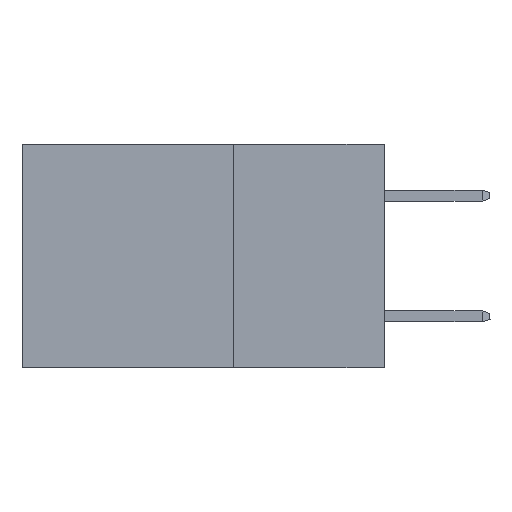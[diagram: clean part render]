
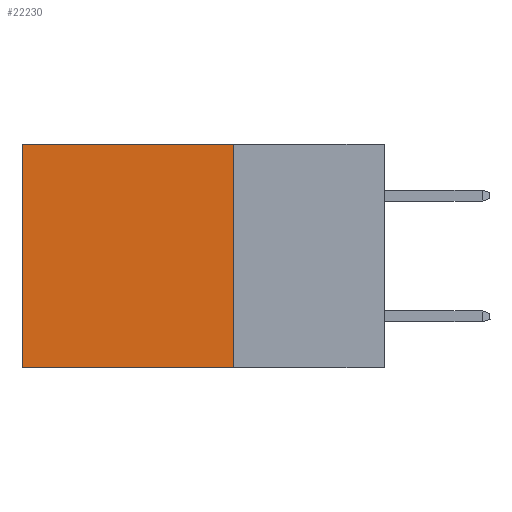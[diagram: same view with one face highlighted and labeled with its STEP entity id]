
A CAD part, left-side view. The second image highlights one B-rep face of the part: STEP entity #22230.
In plain terms, the highlighted planar face has unit normal (-1, 0, 0).
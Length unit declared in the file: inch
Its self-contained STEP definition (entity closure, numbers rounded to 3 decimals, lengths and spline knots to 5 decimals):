
#324 = CARTESIAN_POINT ( 'NONE',  ( 0.2615, 0.6, -0.37 ) ) ;
#365 = EDGE_LOOP ( 'NONE', ( #869, #15367, #24436, #25030 ) ) ;
#869 = ORIENTED_EDGE ( 'NONE', *, *, #14930, .T. ) ;
#1319 = CARTESIAN_POINT ( 'NONE',  ( 0.2615, 0.25, 0. ) ) ;
#2279 = LINE ( 'NONE', #3598, #12925 ) ;
#3598 = CARTESIAN_POINT ( 'NONE',  ( 0.2615, 0.25, -0.37 ) ) ;
#3680 = CARTESIAN_POINT ( 'NONE',  ( 0.2615, 0.25, 0. ) ) ;
#3895 = EDGE_CURVE ( 'NONE', #20038, #16957, #24164, .T. ) ;
#4118 = DIRECTION ( 'NONE',  ( 0., 0., -1. ) ) ;
#4498 = VECTOR ( 'NONE', #7657, 39.37008 ) ;
#4913 = CARTESIAN_POINT ( 'NONE',  ( 0.2615, 0.25, -0.37 ) ) ;
#5964 = VECTOR ( 'NONE', #4118, 39.37008 ) ;
#7657 = DIRECTION ( 'NONE',  ( 0., 1., 0. ) ) ;
#10347 = EDGE_CURVE ( 'NONE', #20038, #16766, #26864, .T. ) ;
#10681 = CARTESIAN_POINT ( 'NONE',  ( 0.2615, 0.25, -0.37 ) ) ;
#11601 = LINE ( 'NONE', #21002, #5964 ) ;
#12494 = DIRECTION ( 'NONE',  ( 0., 0., -1. ) ) ;
#12925 = VECTOR ( 'NONE', #22610, 39.37008 ) ;
#13458 = DIRECTION ( 'NONE',  ( 0., 0., -1. ) ) ;
#14129 = EDGE_CURVE ( 'NONE', #16957, #21756, #2279, .T. ) ;
#14930 = EDGE_CURVE ( 'NONE', #16766, #21756, #11601, .T. ) ;
#15367 = ORIENTED_EDGE ( 'NONE', *, *, #14129, .F. ) ;
#16766 = VERTEX_POINT ( 'NONE', #18459 ) ;
#16957 = VERTEX_POINT ( 'NONE', #10681 ) ;
#18459 = CARTESIAN_POINT ( 'NONE',  ( 0.2615, 0.6, 0. ) ) ;
#18626 = VECTOR ( 'NONE', #13458, 39.37008 ) ;
#19503 = FACE_OUTER_BOUND ( 'NONE', #365, .T. ) ;
#20038 = VERTEX_POINT ( 'NONE', #3680 ) ;
#20826 = PLANE ( 'NONE',  #21003 ) ;
#21002 = CARTESIAN_POINT ( 'NONE',  ( 0.2615, 0.6, -0.37 ) ) ;
#21003 = AXIS2_PLACEMENT_3D ( 'NONE', #22959, #25022, #12494 ) ;
#21756 = VERTEX_POINT ( 'NONE', #324 ) ;
#22230 = ADVANCED_FACE ( 'NONE', ( #19503 ), #20826, .F. ) ;
#22610 = DIRECTION ( 'NONE',  ( 0., 1., 0. ) ) ;
#22959 = CARTESIAN_POINT ( 'NONE',  ( 0.2615, 0.25, -0.37 ) ) ;
#24164 = LINE ( 'NONE', #4913, #18626 ) ;
#24436 = ORIENTED_EDGE ( 'NONE', *, *, #3895, .F. ) ;
#25022 = DIRECTION ( 'NONE',  ( 1., 0., 0. ) ) ;
#25030 = ORIENTED_EDGE ( 'NONE', *, *, #10347, .T. ) ;
#26864 = LINE ( 'NONE', #1319, #4498 ) ;
